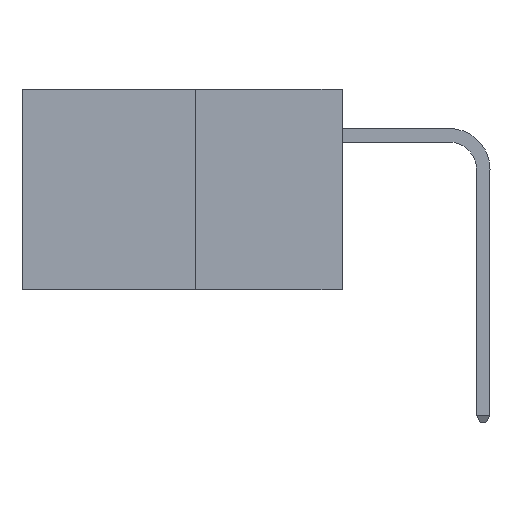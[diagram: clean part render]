
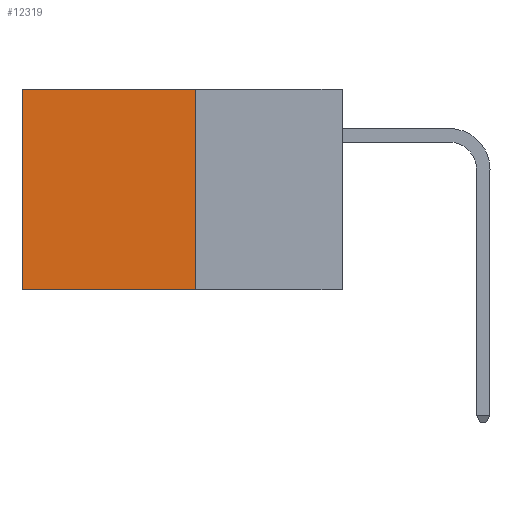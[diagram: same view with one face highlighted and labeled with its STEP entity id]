
A CAD part, left-side view. The second image highlights one B-rep face of the part: STEP entity #12319.
In plain terms, the highlighted planar face has unit normal (-1, 0, 0).
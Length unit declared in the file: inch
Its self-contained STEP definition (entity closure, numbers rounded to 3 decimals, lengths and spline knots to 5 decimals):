
#59 = CARTESIAN_POINT ( 'NONE',  ( 0.277, 0.27, 0. ) ) ;
#1008 = CARTESIAN_POINT ( 'NONE',  ( 0.277, 0.59, -0.37 ) ) ;
#1255 = EDGE_CURVE ( 'NONE', #16970, #3601, #18277, .T. ) ;
#1590 = FACE_OUTER_BOUND ( 'NONE', #7270, .T. ) ;
#1789 = ORIENTED_EDGE ( 'NONE', *, *, #1255, .F. ) ;
#2624 = DIRECTION ( 'NONE',  ( 0., 0., -1. ) ) ;
#2751 = CARTESIAN_POINT ( 'NONE',  ( 0.277, 0.59, 0. ) ) ;
#3601 = VERTEX_POINT ( 'NONE', #12813 ) ;
#3771 = VECTOR ( 'NONE', #2624, 39.37008 ) ;
#3939 = CARTESIAN_POINT ( 'NONE',  ( 0.277, 0.27, 0. ) ) ;
#4544 = EDGE_CURVE ( 'NONE', #3601, #15266, #8808, .T. ) ;
#4585 = VECTOR ( 'NONE', #19982, 39.37008 ) ;
#6082 = AXIS2_PLACEMENT_3D ( 'NONE', #6675, #19504, #9883 ) ;
#6189 = ORIENTED_EDGE ( 'NONE', *, *, #8623, .T. ) ;
#6675 = CARTESIAN_POINT ( 'NONE',  ( 0.277, 0.27, -0.37 ) ) ;
#7270 = EDGE_LOOP ( 'NONE', ( #6189, #10563, #1789, #15538 ) ) ;
#7363 = VERTEX_POINT ( 'NONE', #2751 ) ;
#7931 = CARTESIAN_POINT ( 'NONE',  ( 0.277, 0.27, -0.37 ) ) ;
#8623 = EDGE_CURVE ( 'NONE', #7363, #15266, #12771, .T. ) ;
#8808 = LINE ( 'NONE', #7931, #4585 ) ;
#8919 = EDGE_CURVE ( 'NONE', #16970, #7363, #19072, .T. ) ;
#9883 = DIRECTION ( 'NONE',  ( 0., 0., -1. ) ) ;
#10504 = VECTOR ( 'NONE', #11297, 39.37008 ) ;
#10563 = ORIENTED_EDGE ( 'NONE', *, *, #4544, .F. ) ;
#11297 = DIRECTION ( 'NONE',  ( 0., 1., 0. ) ) ;
#12319 = ADVANCED_FACE ( 'NONE', ( #1590 ), #17917, .F. ) ;
#12771 = LINE ( 'NONE', #1008, #3771 ) ;
#12813 = CARTESIAN_POINT ( 'NONE',  ( 0.277, 0.27, -0.37 ) ) ;
#13959 = VECTOR ( 'NONE', #15477, 39.37008 ) ;
#15107 = CARTESIAN_POINT ( 'NONE',  ( 0.277, 0.59, -0.37 ) ) ;
#15266 = VERTEX_POINT ( 'NONE', #15107 ) ;
#15477 = DIRECTION ( 'NONE',  ( 0., 0., -1. ) ) ;
#15538 = ORIENTED_EDGE ( 'NONE', *, *, #8919, .T. ) ;
#15785 = CARTESIAN_POINT ( 'NONE',  ( 0.277, 0.27, -0.37 ) ) ;
#16970 = VERTEX_POINT ( 'NONE', #3939 ) ;
#17917 = PLANE ( 'NONE',  #6082 ) ;
#18277 = LINE ( 'NONE', #15785, #13959 ) ;
#19072 = LINE ( 'NONE', #59, #10504 ) ;
#19504 = DIRECTION ( 'NONE',  ( 1., 0., 0. ) ) ;
#19982 = DIRECTION ( 'NONE',  ( 0., 1., 0. ) ) ;
